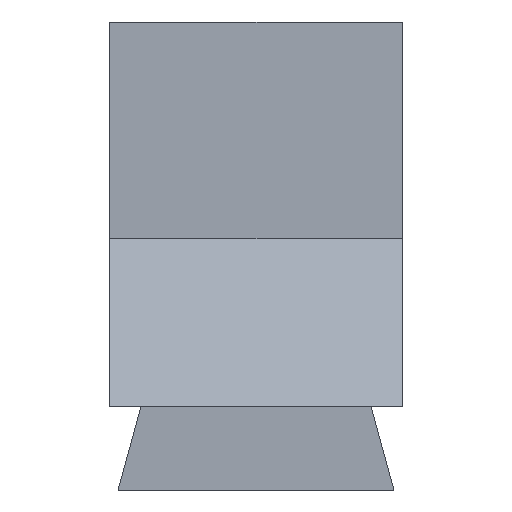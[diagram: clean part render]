
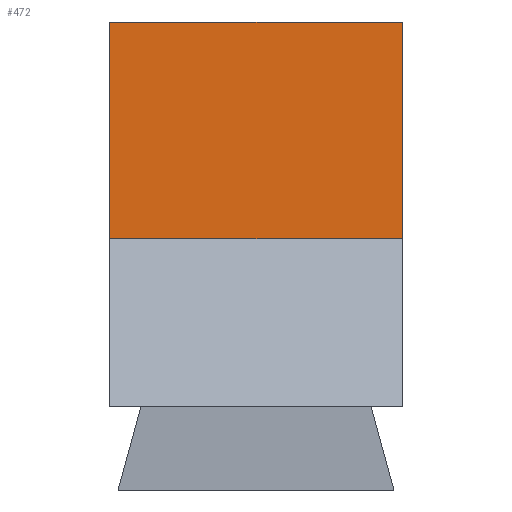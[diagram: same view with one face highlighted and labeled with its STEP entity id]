
A CAD part, left-side view. The second image highlights one B-rep face of the part: STEP entity #472.
In plain terms, the highlighted planar face has unit normal (-1, 0, 0).
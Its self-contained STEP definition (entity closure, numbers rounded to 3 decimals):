
#40 = VERTEX_POINT('',#41);
#41 = CARTESIAN_POINT('',(-6.5,-3.5,4.005));
#119 = EDGE_CURVE('',#40,#120,#122,.T.);
#120 = VERTEX_POINT('',#121);
#121 = CARTESIAN_POINT('',(-6.5,-3.5,9.2));
#122 = LINE('',#123,#124);
#123 = CARTESIAN_POINT('',(-6.5,-3.5,0.));
#124 = VECTOR('',#125,1.);
#125 = DIRECTION('',(0.,0.,1.));
#253 = VERTEX_POINT('',#254);
#254 = CARTESIAN_POINT('',(-6.5,3.5,4.005));
#278 = EDGE_CURVE('',#40,#253,#279,.T.);
#279 = LINE('',#280,#281);
#280 = CARTESIAN_POINT('',(-6.5,-3.5,4.005));
#281 = VECTOR('',#282,1.);
#282 = DIRECTION('',(0.,1.,0.));
#453 = VERTEX_POINT('',#454);
#454 = CARTESIAN_POINT('',(-6.5,3.5,9.2));
#460 = EDGE_CURVE('',#120,#453,#461,.T.);
#461 = LINE('',#462,#463);
#462 = CARTESIAN_POINT('',(-6.5,-3.5,9.2));
#463 = VECTOR('',#464,1.);
#464 = DIRECTION('',(0.,1.,0.));
#472 = ADVANCED_FACE('',(#473),#484,.F.);
#473 = FACE_BOUND('',#474,.F.);
#474 = EDGE_LOOP('',(#475,#476,#477,#483));
#475 = ORIENTED_EDGE('',*,*,#119,.F.);
#476 = ORIENTED_EDGE('',*,*,#278,.T.);
#477 = ORIENTED_EDGE('',*,*,#478,.T.);
#478 = EDGE_CURVE('',#253,#453,#479,.T.);
#479 = LINE('',#480,#481);
#480 = CARTESIAN_POINT('',(-6.5,3.5,0.));
#481 = VECTOR('',#482,1.);
#482 = DIRECTION('',(0.,0.,1.));
#483 = ORIENTED_EDGE('',*,*,#460,.F.);
#484 = PLANE('',#485);
#485 = AXIS2_PLACEMENT_3D('',#486,#487,#488);
#486 = CARTESIAN_POINT('',(-6.5,-3.5,0.));
#487 = DIRECTION('',(1.,0.,0.));
#488 = DIRECTION('',(0.,0.,1.));
